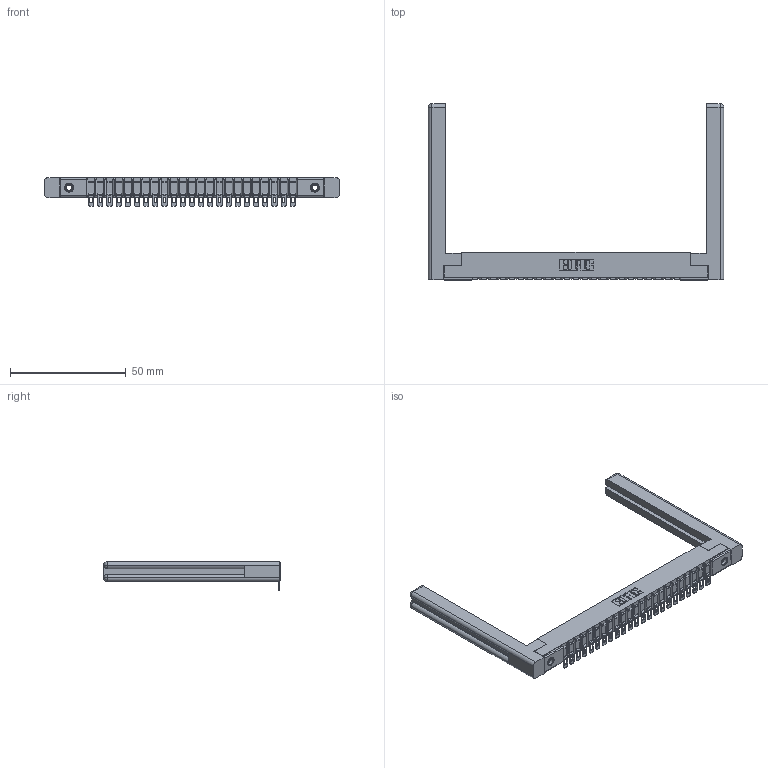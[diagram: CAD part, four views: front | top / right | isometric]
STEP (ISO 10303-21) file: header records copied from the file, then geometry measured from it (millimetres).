
FILE_DESCRIPTION (( 'STEP AP203' ), '1' );
FILE_NAME ('357-023-554-158.STEP', '2019-09-16T23:51:29', ( '' ), ( '' ), 'SwSTEP 2.0', 'SolidWorks 2016', '' );
FILE_SCHEMA (( 'CONFIG_CONTROL_DESIGN' ));
Length unit declared in the file: inch
Products named in the file (5): 307-220-058; 307 Part_.156 Dia Mounting Holes; 357-023-554-158; 345-250-001_345-250-001-102; 307-290-002_554
Assembly tree (28 placements, depth 2):
  357-023-554-158
    307 Part_.156 Dia Mounting Holes
    307-290-002_554  x23
    307-220-058  x2
    345-250-001_345-250-001-102  x2
Bounding box: 127.76 x 76.33 x 12.52 mm (x, y, z)
Volume: 16121.8 mm3; surface area: 20531.7 mm2
Topology: 28 solids, 28 shells, 2147 faces, 6496 edges, 4252 vertices
Faces by surface type: plane 1212, cylinder 863, sphere 48, torus 12, cone 12
Entity records: 25658 total; most frequent: CARTESIAN_POINT 4333, ORIENTED_EDGE 4262, DIRECTION 4185, EDGE_CURVE 2131, LINE 1613, VECTOR 1613, VERTEX_POINT 1380, AXIS2_PLACEMENT_3D 1286
